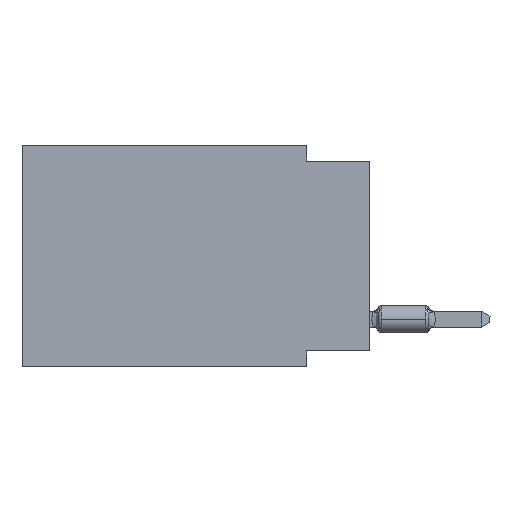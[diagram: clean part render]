
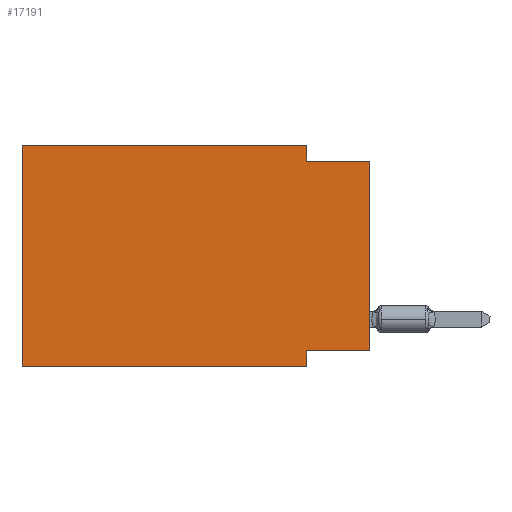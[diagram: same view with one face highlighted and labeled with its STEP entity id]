
A CAD part, left-side view. The second image highlights one B-rep face of the part: STEP entity #17191.
In plain terms, the highlighted planar face has unit normal (-1, 0, 0).
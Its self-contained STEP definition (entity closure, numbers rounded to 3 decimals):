
#14 = FACE_OUTER_BOUND ( 'NONE', #22011, .T. ) ;
#137 = CARTESIAN_POINT ( 'NONE',  ( 0., 13.97, 0. ) ) ;
#670 = LINE ( 'NONE', #14322, #1883 ) ;
#681 = VECTOR ( 'NONE', #10654, 1000. ) ;
#1733 = LINE ( 'NONE', #13565, #4136 ) ;
#1791 = AXIS2_PLACEMENT_3D ( 'NONE', #137, #25326, #6047 ) ;
#1883 = VECTOR ( 'NONE', #22142, 1000. ) ;
#2443 = ORIENTED_EDGE ( 'NONE', *, *, #21058, .F. ) ;
#2516 = EDGE_CURVE ( 'NONE', #24817, #14597, #670, .T. ) ;
#3578 = CARTESIAN_POINT ( 'NONE',  ( 0., 13.97, 0. ) ) ;
#4136 = VECTOR ( 'NONE', #5332, 1000. ) ;
#4319 = DIRECTION ( 'NONE',  ( 0., 1., 0. ) ) ;
#4907 = ORIENTED_EDGE ( 'NONE', *, *, #10462, .F. ) ;
#4919 = CARTESIAN_POINT ( 'NONE',  ( 0., 13.97, -8.89 ) ) ;
#5332 = DIRECTION ( 'NONE',  ( 0., -1., 0. ) ) ;
#5389 = VECTOR ( 'NONE', #22599, 1000. ) ;
#6047 = DIRECTION ( 'NONE',  ( 0., 0., -1. ) ) ;
#6917 = CARTESIAN_POINT ( 'NONE',  ( 0., 2.54, -8.89 ) ) ;
#7362 = EDGE_CURVE ( 'NONE', #8948, #7394, #14412, .T. ) ;
#7394 = VERTEX_POINT ( 'NONE', #7871 ) ;
#7674 = CARTESIAN_POINT ( 'NONE',  ( 0., 0., 0. ) ) ;
#7871 = CARTESIAN_POINT ( 'NONE',  ( 0., 0., -0.635 ) ) ;
#8188 = VECTOR ( 'NONE', #11749, 1000. ) ;
#8948 = VERTEX_POINT ( 'NONE', #20298 ) ;
#8990 = EDGE_CURVE ( 'NONE', #14795, #11585, #20549, .T. ) ;
#9915 = PLANE ( 'NONE',  #1791 ) ;
#10462 = EDGE_CURVE ( 'NONE', #13008, #14795, #12307, .T. ) ;
#10654 = DIRECTION ( 'NONE',  ( 0., 0., 1. ) ) ;
#10908 = CARTESIAN_POINT ( 'NONE',  ( 0., 13.97, 0. ) ) ;
#10990 = ORIENTED_EDGE ( 'NONE', *, *, #14414, .T. ) ;
#11084 = ORIENTED_EDGE ( 'NONE', *, *, #2516, .F. ) ;
#11107 = CARTESIAN_POINT ( 'NONE',  ( 0., 2.54, -8.255 ) ) ;
#11559 = LINE ( 'NONE', #7674, #22981 ) ;
#11570 = EDGE_CURVE ( 'NONE', #13008, #7394, #11559, .T. ) ;
#11585 = VERTEX_POINT ( 'NONE', #21426 ) ;
#11749 = DIRECTION ( 'NONE',  ( 0., -1., 0. ) ) ;
#11784 = ORIENTED_EDGE ( 'NONE', *, *, #7362, .F. ) ;
#11899 = EDGE_CURVE ( 'NONE', #14597, #8948, #20906, .T. ) ;
#12307 = LINE ( 'NONE', #14103, #15988 ) ;
#12435 = VERTEX_POINT ( 'NONE', #4919 ) ;
#13008 = VERTEX_POINT ( 'NONE', #15641 ) ;
#13565 = CARTESIAN_POINT ( 'NONE',  ( 0., 13.97, -8.89 ) ) ;
#13610 = DIRECTION ( 'NONE',  ( 0., 0., 1. ) ) ;
#13968 = VECTOR ( 'NONE', #16936, 1000. ) ;
#14103 = CARTESIAN_POINT ( 'NONE',  ( 0., 0., -8.255 ) ) ;
#14322 = CARTESIAN_POINT ( 'NONE',  ( 0., 13.97, 0. ) ) ;
#14412 = LINE ( 'NONE', #16341, #8188 ) ;
#14414 = EDGE_CURVE ( 'NONE', #12435, #11585, #1733, .T. ) ;
#14597 = VERTEX_POINT ( 'NONE', #17797 ) ;
#14770 = LINE ( 'NONE', #10908, #681 ) ;
#14795 = VERTEX_POINT ( 'NONE', #11107 ) ;
#14885 = CARTESIAN_POINT ( 'NONE',  ( 0., 2.54, 0. ) ) ;
#15641 = CARTESIAN_POINT ( 'NONE',  ( 0., 0., -8.255 ) ) ;
#15988 = VECTOR ( 'NONE', #4319, 1000. ) ;
#16341 = CARTESIAN_POINT ( 'NONE',  ( 0., 0., -0.635 ) ) ;
#16936 = DIRECTION ( 'NONE',  ( 0., 0., -1. ) ) ;
#17191 = ADVANCED_FACE ( 'NONE', ( #14 ), #9915, .F. ) ;
#17403 = ORIENTED_EDGE ( 'NONE', *, *, #8990, .F. ) ;
#17656 = ORIENTED_EDGE ( 'NONE', *, *, #11570, .T. ) ;
#17797 = CARTESIAN_POINT ( 'NONE',  ( 0., 2.54, 0. ) ) ;
#20298 = CARTESIAN_POINT ( 'NONE',  ( 0., 2.54, -0.635 ) ) ;
#20549 = LINE ( 'NONE', #6917, #5389 ) ;
#20906 = LINE ( 'NONE', #14885, #13968 ) ;
#21058 = EDGE_CURVE ( 'NONE', #12435, #24817, #14770, .T. ) ;
#21426 = CARTESIAN_POINT ( 'NONE',  ( 0., 2.54, -8.89 ) ) ;
#22011 = EDGE_LOOP ( 'NONE', ( #17656, #11784, #24317, #11084, #2443, #10990, #17403, #4907 ) ) ;
#22142 = DIRECTION ( 'NONE',  ( 0., -1., 0. ) ) ;
#22599 = DIRECTION ( 'NONE',  ( 0., 0., -1. ) ) ;
#22981 = VECTOR ( 'NONE', #13610, 1000. ) ;
#24317 = ORIENTED_EDGE ( 'NONE', *, *, #11899, .F. ) ;
#24817 = VERTEX_POINT ( 'NONE', #3578 ) ;
#25326 = DIRECTION ( 'NONE',  ( 1., 0., 0. ) ) ;
